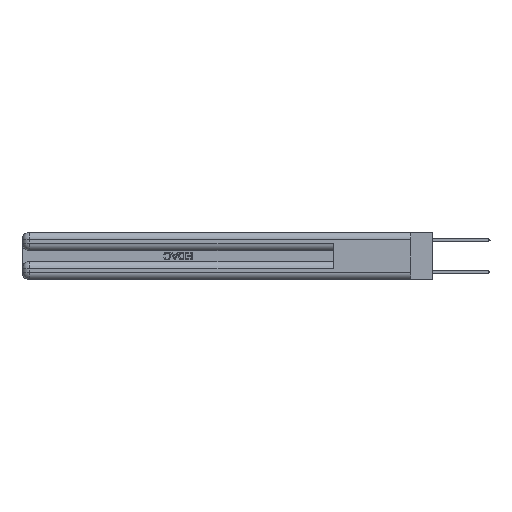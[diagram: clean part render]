
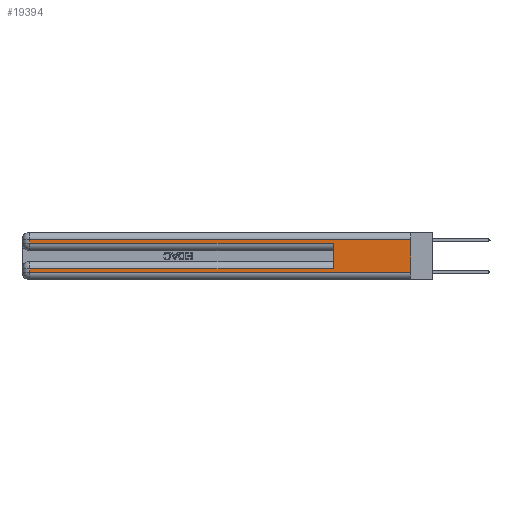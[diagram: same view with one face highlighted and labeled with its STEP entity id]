
A CAD part, left-side view. The second image highlights one B-rep face of the part: STEP entity #19394.
In plain terms, the highlighted planar face has unit normal (-1, 0, 0).
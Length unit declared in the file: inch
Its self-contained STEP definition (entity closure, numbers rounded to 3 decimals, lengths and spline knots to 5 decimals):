
#395 = VECTOR ( 'NONE', #19482, 39.37008 ) ;
#751 = CARTESIAN_POINT ( 'NONE',  ( 0., 0., 0.37 ) ) ;
#1323 = VECTOR ( 'NONE', #25961, 39.37008 ) ;
#1356 = LINE ( 'NONE', #23175, #24164 ) ;
#1900 = DIRECTION ( 'NONE',  ( 0., 0., 1. ) ) ;
#2765 = LINE ( 'NONE', #23261, #17139 ) ;
#3274 = DIRECTION ( 'NONE',  ( 0., 1., 0. ) ) ;
#3656 = PLANE ( 'NONE',  #25394 ) ;
#3925 = EDGE_LOOP ( 'NONE', ( #36540, #33673, #10055, #10822, #14607, #15888, #5399, #26376 ) ) ;
#4018 = EDGE_CURVE ( 'NONE', #5095, #29125, #34463, .T. ) ;
#4745 = CARTESIAN_POINT ( 'NONE',  ( 0., 0., 0.285 ) ) ;
#5095 = VERTEX_POINT ( 'NONE', #30940 ) ;
#5399 = ORIENTED_EDGE ( 'NONE', *, *, #18922, .T. ) ;
#5776 = DIRECTION ( 'NONE',  ( 0., 1., 0. ) ) ;
#6084 = DIRECTION ( 'NONE',  ( 0., 0., -1. ) ) ;
#6446 = EDGE_CURVE ( 'NONE', #28226, #18134, #2765, .T. ) ;
#6541 = DIRECTION ( 'NONE',  ( 0., 0., -1. ) ) ;
#7837 = VERTEX_POINT ( 'NONE', #23055 ) ;
#7855 = EDGE_CURVE ( 'NONE', #18134, #5095, #1356, .T. ) ;
#8352 = EDGE_CURVE ( 'NONE', #28226, #29295, #8935, .T. ) ;
#8935 = LINE ( 'NONE', #23114, #1323 ) ;
#9091 = VECTOR ( 'NONE', #1900, 39.37008 ) ;
#10028 = EDGE_CURVE ( 'NONE', #24820, #15410, #29357, .T. ) ;
#10055 = ORIENTED_EDGE ( 'NONE', *, *, #7855, .T. ) ;
#10822 = ORIENTED_EDGE ( 'NONE', *, *, #4018, .T. ) ;
#10970 = CARTESIAN_POINT ( 'NONE',  ( 0., 0., 0.06 ) ) ;
#12190 = DIRECTION ( 'NONE',  ( 1., 0., 0. ) ) ;
#14607 = ORIENTED_EDGE ( 'NONE', *, *, #30581, .F. ) ;
#15410 = VERTEX_POINT ( 'NONE', #22033 ) ;
#15888 = ORIENTED_EDGE ( 'NONE', *, *, #10028, .T. ) ;
#16535 = LINE ( 'NONE', #35550, #30738 ) ;
#17139 = VECTOR ( 'NONE', #3274, 39.37008 ) ;
#18134 = VERTEX_POINT ( 'NONE', #32154 ) ;
#18922 = EDGE_CURVE ( 'NONE', #15410, #7837, #16535, .T. ) ;
#19047 = CARTESIAN_POINT ( 'NONE',  ( 0., 0.6, 0.145 ) ) ;
#19392 = VECTOR ( 'NONE', #33211, 39.37008 ) ;
#19394 = ADVANCED_FACE ( 'NONE', ( #30705 ), #3656, .F. ) ;
#19405 = LINE ( 'NONE', #19047, #9091 ) ;
#19482 = DIRECTION ( 'NONE',  ( 0., -1., 0. ) ) ;
#21264 = CARTESIAN_POINT ( 'NONE',  ( 0., 0., 0.06 ) ) ;
#21450 = DIRECTION ( 'NONE',  ( 0., 0., -1. ) ) ;
#22033 = CARTESIAN_POINT ( 'NONE',  ( 0., 2.94, 0.085 ) ) ;
#22685 = VECTOR ( 'NONE', #5776, 39.37008 ) ;
#23055 = CARTESIAN_POINT ( 'NONE',  ( 0., 2.94, 0.06 ) ) ;
#23114 = CARTESIAN_POINT ( 'NONE',  ( 0., 0., 0.37 ) ) ;
#23175 = CARTESIAN_POINT ( 'NONE',  ( 0., 2.94, 0.37 ) ) ;
#23243 = LINE ( 'NONE', #10970, #395 ) ;
#23261 = CARTESIAN_POINT ( 'NONE',  ( 0., 0., 0.31 ) ) ;
#24164 = VECTOR ( 'NONE', #6084, 39.37008 ) ;
#24820 = VERTEX_POINT ( 'NONE', #31201 ) ;
#25394 = AXIS2_PLACEMENT_3D ( 'NONE', #751, #12190, #6541 ) ;
#25961 = DIRECTION ( 'NONE',  ( 0., 0., -1. ) ) ;
#26376 = ORIENTED_EDGE ( 'NONE', *, *, #36021, .T. ) ;
#26419 = CARTESIAN_POINT ( 'NONE',  ( 0., 0., 0.31 ) ) ;
#28226 = VERTEX_POINT ( 'NONE', #26419 ) ;
#28587 = CARTESIAN_POINT ( 'NONE',  ( 0., 0., 0.085 ) ) ;
#29125 = VERTEX_POINT ( 'NONE', #31940 ) ;
#29295 = VERTEX_POINT ( 'NONE', #21264 ) ;
#29357 = LINE ( 'NONE', #28587, #22685 ) ;
#30581 = EDGE_CURVE ( 'NONE', #24820, #29125, #19405, .T. ) ;
#30705 = FACE_OUTER_BOUND ( 'NONE', #3925, .T. ) ;
#30738 = VECTOR ( 'NONE', #21450, 39.37008 ) ;
#30940 = CARTESIAN_POINT ( 'NONE',  ( 0., 2.94, 0.285 ) ) ;
#31201 = CARTESIAN_POINT ( 'NONE',  ( 0., 0.6, 0.085 ) ) ;
#31940 = CARTESIAN_POINT ( 'NONE',  ( 0., 0.6, 0.285 ) ) ;
#32154 = CARTESIAN_POINT ( 'NONE',  ( 0., 2.94, 0.31 ) ) ;
#33211 = DIRECTION ( 'NONE',  ( 0., -1., 0. ) ) ;
#33673 = ORIENTED_EDGE ( 'NONE', *, *, #6446, .T. ) ;
#34463 = LINE ( 'NONE', #4745, #19392 ) ;
#35550 = CARTESIAN_POINT ( 'NONE',  ( 0., 2.94, 0.37 ) ) ;
#36021 = EDGE_CURVE ( 'NONE', #7837, #29295, #23243, .T. ) ;
#36540 = ORIENTED_EDGE ( 'NONE', *, *, #8352, .F. ) ;
